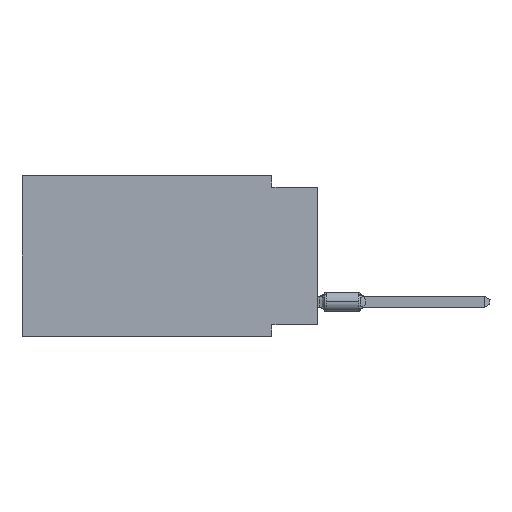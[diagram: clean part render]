
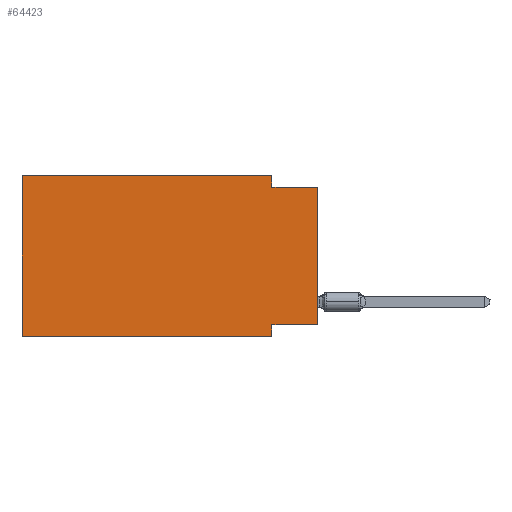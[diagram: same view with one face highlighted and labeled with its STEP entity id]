
A CAD part, left-side view. The second image highlights one B-rep face of the part: STEP entity #64423.
In plain terms, the highlighted planar face has unit normal (-1, 0, 0).
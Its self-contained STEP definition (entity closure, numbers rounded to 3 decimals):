
#807 = LINE ( 'NONE', #21873, #68182 ) ;
#980 = CARTESIAN_POINT ( 'NONE',  ( 0., 16.383, 0. ) ) ;
#2614 = CARTESIAN_POINT ( 'NONE',  ( 0., 16.383, -8.89 ) ) ;
#2675 = VERTEX_POINT ( 'NONE', #77608 ) ;
#4158 = CARTESIAN_POINT ( 'NONE',  ( 0., 16.383, 0. ) ) ;
#4229 = DIRECTION ( 'NONE',  ( 0., 0., -1. ) ) ;
#4609 = LINE ( 'NONE', #4158, #31209 ) ;
#5049 = ORIENTED_EDGE ( 'NONE', *, *, #29182, .F. ) ;
#8417 = CARTESIAN_POINT ( 'NONE',  ( 0., 2.54, 0. ) ) ;
#11257 = ORIENTED_EDGE ( 'NONE', *, *, #82763, .T. ) ;
#13021 = VECTOR ( 'NONE', #75015, 1000. ) ;
#16416 = VECTOR ( 'NONE', #22033, 1000. ) ;
#18653 = CARTESIAN_POINT ( 'NONE',  ( 0., 2.54, -8.89 ) ) ;
#19297 = DIRECTION ( 'NONE',  ( 0., -1., 0. ) ) ;
#19343 = LINE ( 'NONE', #67413, #64580 ) ;
#21222 = VERTEX_POINT ( 'NONE', #26002 ) ;
#21394 = VERTEX_POINT ( 'NONE', #35952 ) ;
#21873 = CARTESIAN_POINT ( 'NONE',  ( 0., 0., 0. ) ) ;
#22033 = DIRECTION ( 'NONE',  ( 0., 0., -1. ) ) ;
#22673 = DIRECTION ( 'NONE',  ( 0., 1., 0. ) ) ;
#26002 = CARTESIAN_POINT ( 'NONE',  ( 0., 2.54, -0.635 ) ) ;
#27731 = EDGE_LOOP ( 'NONE', ( #11257, #31401, #85425, #5049, #48847, #86680, #47116, #57451 ) ) ;
#28812 = DIRECTION ( 'NONE',  ( 0., 0., -1. ) ) ;
#29182 = EDGE_CURVE ( 'NONE', #2675, #43641, #78810, .T. ) ;
#29283 = EDGE_CURVE ( 'NONE', #61556, #2675, #4609, .T. ) ;
#29821 = DIRECTION ( 'NONE',  ( 0., -1., 0. ) ) ;
#31209 = VECTOR ( 'NONE', #52689, 1000. ) ;
#31401 = ORIENTED_EDGE ( 'NONE', *, *, #43018, .F. ) ;
#33807 = EDGE_CURVE ( 'NONE', #21394, #35157, #35474, .T. ) ;
#35157 = VERTEX_POINT ( 'NONE', #69098 ) ;
#35474 = LINE ( 'NONE', #69846, #71031 ) ;
#35952 = CARTESIAN_POINT ( 'NONE',  ( 0., 0., -8.255 ) ) ;
#36567 = DIRECTION ( 'NONE',  ( 1., 0., 0. ) ) ;
#36682 = CARTESIAN_POINT ( 'NONE',  ( 0., 0., -0.635 ) ) ;
#42536 = PLANE ( 'NONE',  #90420 ) ;
#42882 = VECTOR ( 'NONE', #29821, 1000. ) ;
#43018 = EDGE_CURVE ( 'NONE', #21222, #69887, #75463, .T. ) ;
#43641 = VERTEX_POINT ( 'NONE', #8417 ) ;
#44139 = VECTOR ( 'NONE', #19297, 1000. ) ;
#47116 = ORIENTED_EDGE ( 'NONE', *, *, #76018, .F. ) ;
#47987 = EDGE_CURVE ( 'NONE', #43641, #21222, #51291, .T. ) ;
#48847 = ORIENTED_EDGE ( 'NONE', *, *, #29283, .F. ) ;
#51291 = LINE ( 'NONE', #84750, #16416 ) ;
#52689 = DIRECTION ( 'NONE',  ( 0., 0., 1. ) ) ;
#57451 = ORIENTED_EDGE ( 'NONE', *, *, #33807, .F. ) ;
#57573 = DIRECTION ( 'NONE',  ( 0., 0., 1. ) ) ;
#60047 = LINE ( 'NONE', #60953, #44139 ) ;
#60953 = CARTESIAN_POINT ( 'NONE',  ( 0., 16.383, -8.89 ) ) ;
#61556 = VERTEX_POINT ( 'NONE', #2614 ) ;
#63177 = FACE_OUTER_BOUND ( 'NONE', #27731, .T. ) ;
#64423 = ADVANCED_FACE ( 'NONE', ( #63177 ), #42536, .F. ) ;
#64580 = VECTOR ( 'NONE', #4229, 1000. ) ;
#67413 = CARTESIAN_POINT ( 'NONE',  ( 0., 2.54, -8.89 ) ) ;
#68182 = VECTOR ( 'NONE', #57573, 1000. ) ;
#69098 = CARTESIAN_POINT ( 'NONE',  ( 0., 2.54, -8.255 ) ) ;
#69846 = CARTESIAN_POINT ( 'NONE',  ( 0., 0., -8.255 ) ) ;
#69887 = VERTEX_POINT ( 'NONE', #36682 ) ;
#70855 = EDGE_CURVE ( 'NONE', #61556, #72907, #60047, .T. ) ;
#71031 = VECTOR ( 'NONE', #22673, 1000. ) ;
#72907 = VERTEX_POINT ( 'NONE', #18653 ) ;
#75015 = DIRECTION ( 'NONE',  ( 0., -1., 0. ) ) ;
#75463 = LINE ( 'NONE', #88312, #13021 ) ;
#76018 = EDGE_CURVE ( 'NONE', #35157, #72907, #19343, .T. ) ;
#77608 = CARTESIAN_POINT ( 'NONE',  ( 0., 16.383, 0. ) ) ;
#78810 = LINE ( 'NONE', #980, #42882 ) ;
#82763 = EDGE_CURVE ( 'NONE', #21394, #69887, #807, .T. ) ;
#84750 = CARTESIAN_POINT ( 'NONE',  ( 0., 2.54, 0. ) ) ;
#85425 = ORIENTED_EDGE ( 'NONE', *, *, #47987, .F. ) ;
#86033 = CARTESIAN_POINT ( 'NONE',  ( 0., 16.383, 0. ) ) ;
#86680 = ORIENTED_EDGE ( 'NONE', *, *, #70855, .T. ) ;
#88312 = CARTESIAN_POINT ( 'NONE',  ( 0., 0., -0.635 ) ) ;
#90420 = AXIS2_PLACEMENT_3D ( 'NONE', #86033, #36567, #28812 ) ;
